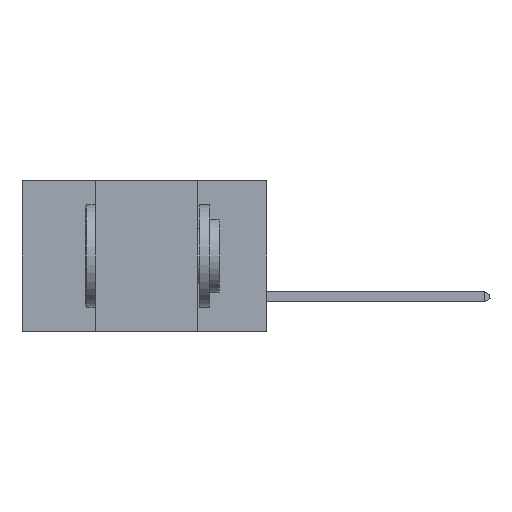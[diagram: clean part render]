
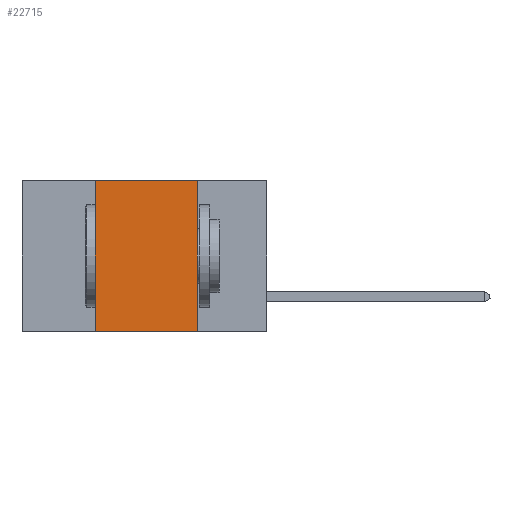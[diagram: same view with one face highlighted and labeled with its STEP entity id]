
A CAD part, left-side view. The second image highlights one B-rep face of the part: STEP entity #22715.
In plain terms, the highlighted planar face has unit normal (-1, 0, 0).
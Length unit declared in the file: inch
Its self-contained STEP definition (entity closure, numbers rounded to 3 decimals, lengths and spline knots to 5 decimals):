
#964 = EDGE_CURVE ( 'NONE', #10255, #13075, #21125, .T. ) ;
#1425 = LINE ( 'NONE', #17931, #6523 ) ;
#2309 = ORIENTED_EDGE ( 'NONE', *, *, #39888, .F. ) ;
#2418 = FACE_OUTER_BOUND ( 'NONE', #42286, .T. ) ;
#3449 = DIRECTION ( 'NONE',  ( 0., -1., 0. ) ) ;
#5134 = DIRECTION ( 'NONE',  ( 1., 0., 0. ) ) ;
#6523 = VECTOR ( 'NONE', #28239, 39.37008 ) ;
#8997 = DIRECTION ( 'NONE',  ( 0., -1., 0. ) ) ;
#9950 = VECTOR ( 'NONE', #8997, 39.37008 ) ;
#10255 = VERTEX_POINT ( 'NONE', #45675 ) ;
#11353 = CARTESIAN_POINT ( 'NONE',  ( 0., 0.17, 0. ) ) ;
#13075 = VERTEX_POINT ( 'NONE', #32390 ) ;
#14492 = CARTESIAN_POINT ( 'NONE',  ( 0., 0.6, -0.37 ) ) ;
#14882 = EDGE_CURVE ( 'NONE', #43546, #13075, #1425, .T. ) ;
#17931 = CARTESIAN_POINT ( 'NONE',  ( 0., 0.17, 0. ) ) ;
#18930 = CARTESIAN_POINT ( 'NONE',  ( 0., 0.6, 0. ) ) ;
#20265 = VERTEX_POINT ( 'NONE', #22255 ) ;
#21125 = LINE ( 'NONE', #14492, #45581 ) ;
#22255 = CARTESIAN_POINT ( 'NONE',  ( 0., 0.42, 0. ) ) ;
#22715 = ADVANCED_FACE ( 'NONE', ( #2418 ), #36696, .F. ) ;
#22789 = CARTESIAN_POINT ( 'NONE',  ( 0., 0.6, 0. ) ) ;
#24379 = LINE ( 'NONE', #27182, #42156 ) ;
#25477 = ORIENTED_EDGE ( 'NONE', *, *, #39299, .F. ) ;
#27182 = CARTESIAN_POINT ( 'NONE',  ( 0., 0.42, 0. ) ) ;
#28239 = DIRECTION ( 'NONE',  ( 0., 0., -1. ) ) ;
#28851 = LINE ( 'NONE', #22789, #9950 ) ;
#32390 = CARTESIAN_POINT ( 'NONE',  ( 0., 0.17, -0.37 ) ) ;
#33702 = AXIS2_PLACEMENT_3D ( 'NONE', #18930, #5134, #37167 ) ;
#36696 = PLANE ( 'NONE',  #33702 ) ;
#37167 = DIRECTION ( 'NONE',  ( 0., 0., -1. ) ) ;
#38759 = ORIENTED_EDGE ( 'NONE', *, *, #964, .T. ) ;
#39286 = ORIENTED_EDGE ( 'NONE', *, *, #14882, .F. ) ;
#39299 = EDGE_CURVE ( 'NONE', #20265, #43546, #28851, .T. ) ;
#39888 = EDGE_CURVE ( 'NONE', #10255, #20265, #24379, .T. ) ;
#41488 = DIRECTION ( 'NONE',  ( 0., 0., 1. ) ) ;
#42156 = VECTOR ( 'NONE', #41488, 39.37008 ) ;
#42286 = EDGE_LOOP ( 'NONE', ( #39286, #25477, #2309, #38759 ) ) ;
#43546 = VERTEX_POINT ( 'NONE', #11353 ) ;
#45581 = VECTOR ( 'NONE', #3449, 39.37008 ) ;
#45675 = CARTESIAN_POINT ( 'NONE',  ( 0., 0.42, -0.37 ) ) ;
